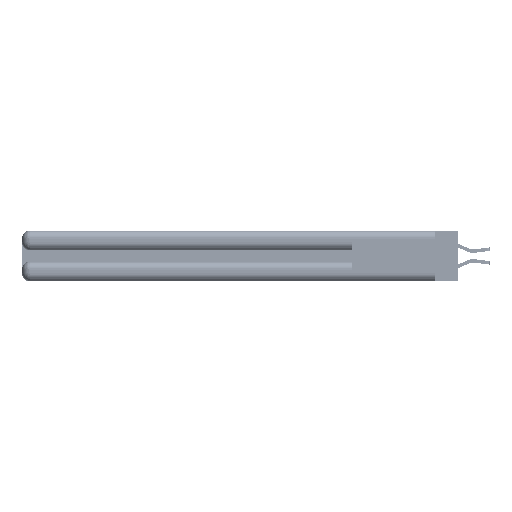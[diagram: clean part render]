
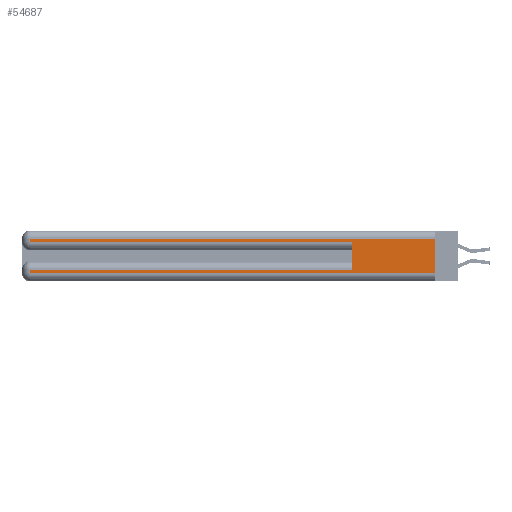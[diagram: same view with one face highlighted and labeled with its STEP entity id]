
A CAD part, left-side view. The second image highlights one B-rep face of the part: STEP entity #54687.
In plain terms, the highlighted planar face has unit normal (-1, 0, 0).
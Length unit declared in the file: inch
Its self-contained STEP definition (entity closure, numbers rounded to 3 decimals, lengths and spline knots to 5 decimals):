
#983 = EDGE_CURVE ( 'NONE', #34650, #25720, #7223, .T. ) ;
#1172 = EDGE_CURVE ( 'NONE', #1388, #27166, #7878, .T. ) ;
#1388 = VERTEX_POINT ( 'NONE', #42660 ) ;
#1940 = LINE ( 'NONE', #26359, #25387 ) ;
#3082 = ORIENTED_EDGE ( 'NONE', *, *, #983, .T. ) ;
#3227 = DIRECTION ( 'NONE',  ( 0., 0., -1. ) ) ;
#3407 = EDGE_CURVE ( 'NONE', #27166, #45502, #11820, .T. ) ;
#4306 = CARTESIAN_POINT ( 'NONE',  ( 0., 0., 0.285 ) ) ;
#5145 = CARTESIAN_POINT ( 'NONE',  ( 0., 0., 0.31 ) ) ;
#7223 = LINE ( 'NONE', #53557, #27877 ) ;
#7878 = LINE ( 'NONE', #10792, #53146 ) ;
#8284 = VECTOR ( 'NONE', #8785, 39.37008 ) ;
#8785 = DIRECTION ( 'NONE',  ( 0., 0., -1. ) ) ;
#9312 = EDGE_CURVE ( 'NONE', #31307, #52362, #42393, .T. ) ;
#10792 = CARTESIAN_POINT ( 'NONE',  ( 0., 0., 0.085 ) ) ;
#10950 = ORIENTED_EDGE ( 'NONE', *, *, #25407, .F. ) ;
#11820 = LINE ( 'NONE', #34000, #22144 ) ;
#12075 = ORIENTED_EDGE ( 'NONE', *, *, #29494, .T. ) ;
#16403 = ORIENTED_EDGE ( 'NONE', *, *, #9312, .T. ) ;
#17610 = DIRECTION ( 'NONE',  ( 0., -1., 0. ) ) ;
#19350 = ORIENTED_EDGE ( 'NONE', *, *, #53141, .T. ) ;
#19521 = DIRECTION ( 'NONE',  ( 1., 0., 0. ) ) ;
#20016 = LINE ( 'NONE', #26330, #8284 ) ;
#20898 = ORIENTED_EDGE ( 'NONE', *, *, #1172, .T. ) ;
#22144 = VECTOR ( 'NONE', #3227, 39.37008 ) ;
#24867 = CARTESIAN_POINT ( 'NONE',  ( 0., 0.6, 0.145 ) ) ;
#25387 = VECTOR ( 'NONE', #34964, 39.37008 ) ;
#25407 = EDGE_CURVE ( 'NONE', #1388, #52362, #38190, .T. ) ;
#25720 = VERTEX_POINT ( 'NONE', #31338 ) ;
#25776 = VECTOR ( 'NONE', #31279, 39.37008 ) ;
#26330 = CARTESIAN_POINT ( 'NONE',  ( 0., 2.94, 0.37 ) ) ;
#26359 = CARTESIAN_POINT ( 'NONE',  ( 0., 0., 0.06 ) ) ;
#26869 = CARTESIAN_POINT ( 'NONE',  ( 0., 0., 0.37 ) ) ;
#27151 = LINE ( 'NONE', #26869, #25776 ) ;
#27166 = VERTEX_POINT ( 'NONE', #49523 ) ;
#27877 = VECTOR ( 'NONE', #40397, 39.37008 ) ;
#28059 = ORIENTED_EDGE ( 'NONE', *, *, #3407, .T. ) ;
#28490 = VERTEX_POINT ( 'NONE', #36657 ) ;
#29270 = DIRECTION ( 'NONE',  ( 0., 0., 1. ) ) ;
#29494 = EDGE_CURVE ( 'NONE', #25720, #31307, #20016, .T. ) ;
#30006 = FACE_OUTER_BOUND ( 'NONE', #41074, .T. ) ;
#30750 = VECTOR ( 'NONE', #17610, 39.37008 ) ;
#31279 = DIRECTION ( 'NONE',  ( 0., 0., -1. ) ) ;
#31307 = VERTEX_POINT ( 'NONE', #42430 ) ;
#31338 = CARTESIAN_POINT ( 'NONE',  ( 0., 2.94, 0.31 ) ) ;
#34000 = CARTESIAN_POINT ( 'NONE',  ( 0., 2.94, 0.37 ) ) ;
#34650 = VERTEX_POINT ( 'NONE', #5145 ) ;
#34964 = DIRECTION ( 'NONE',  ( 0., -1., 0. ) ) ;
#36657 = CARTESIAN_POINT ( 'NONE',  ( 0., 0., 0.06 ) ) ;
#36827 = VECTOR ( 'NONE', #29270, 39.37008 ) ;
#38190 = LINE ( 'NONE', #24867, #36827 ) ;
#40397 = DIRECTION ( 'NONE',  ( 0., 1., 0. ) ) ;
#41074 = EDGE_LOOP ( 'NONE', ( #44159, #3082, #12075, #16403, #10950, #20898, #28059, #19350 ) ) ;
#41402 = PLANE ( 'NONE',  #53866 ) ;
#42393 = LINE ( 'NONE', #4306, #30750 ) ;
#42430 = CARTESIAN_POINT ( 'NONE',  ( 0., 2.94, 0.285 ) ) ;
#42535 = CARTESIAN_POINT ( 'NONE',  ( 0., 0.6, 0.285 ) ) ;
#42660 = CARTESIAN_POINT ( 'NONE',  ( 0., 0.6, 0.085 ) ) ;
#44159 = ORIENTED_EDGE ( 'NONE', *, *, #56342, .F. ) ;
#45502 = VERTEX_POINT ( 'NONE', #51634 ) ;
#45806 = CARTESIAN_POINT ( 'NONE',  ( 0., 0., 0.37 ) ) ;
#45938 = DIRECTION ( 'NONE',  ( 0., 1., 0. ) ) ;
#49523 = CARTESIAN_POINT ( 'NONE',  ( 0., 2.94, 0.085 ) ) ;
#50136 = DIRECTION ( 'NONE',  ( 0., 0., -1. ) ) ;
#51634 = CARTESIAN_POINT ( 'NONE',  ( 0., 2.94, 0.06 ) ) ;
#52362 = VERTEX_POINT ( 'NONE', #42535 ) ;
#53141 = EDGE_CURVE ( 'NONE', #45502, #28490, #1940, .T. ) ;
#53146 = VECTOR ( 'NONE', #45938, 39.37008 ) ;
#53557 = CARTESIAN_POINT ( 'NONE',  ( 0., 0., 0.31 ) ) ;
#53866 = AXIS2_PLACEMENT_3D ( 'NONE', #45806, #19521, #50136 ) ;
#54687 = ADVANCED_FACE ( 'NONE', ( #30006 ), #41402, .F. ) ;
#56342 = EDGE_CURVE ( 'NONE', #34650, #28490, #27151, .T. ) ;
